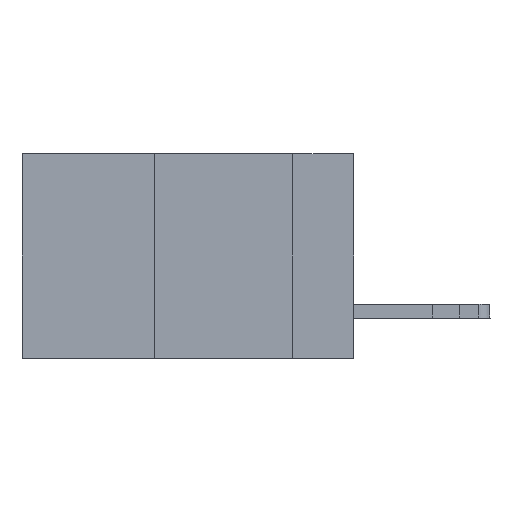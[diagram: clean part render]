
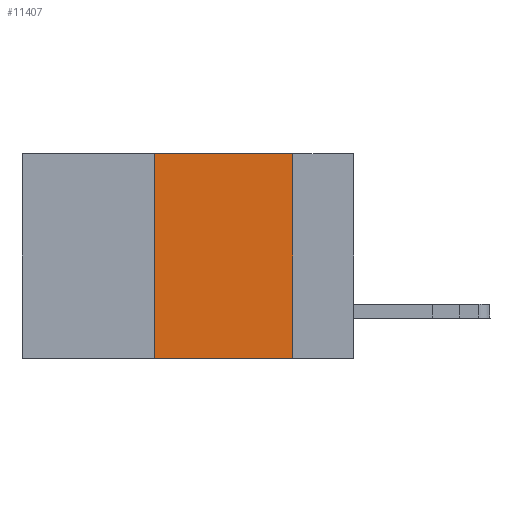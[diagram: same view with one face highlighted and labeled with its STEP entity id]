
A CAD part, left-side view. The second image highlights one B-rep face of the part: STEP entity #11407.
In plain terms, the highlighted planar face has unit normal (-1, 0, 0).
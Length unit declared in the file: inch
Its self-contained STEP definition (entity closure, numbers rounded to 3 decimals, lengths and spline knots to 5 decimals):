
#121 = DIRECTION ( 'NONE',  ( 0., 0., -1. ) ) ;
#979 = CARTESIAN_POINT ( 'NONE',  ( 0., 0.6, -0.37 ) ) ;
#1131 = EDGE_CURVE ( 'NONE', #9691, #8390, #1916, .T. ) ;
#1740 = DIRECTION ( 'NONE',  ( 0., -1., 0. ) ) ;
#1916 = LINE ( 'NONE', #7023, #8599 ) ;
#2719 = DIRECTION ( 'NONE',  ( 0., 0., 1. ) ) ;
#2920 = PLANE ( 'NONE',  #10691 ) ;
#3132 = ORIENTED_EDGE ( 'NONE', *, *, #3309, .F. ) ;
#3309 = EDGE_CURVE ( 'NONE', #19067, #4834, #12117, .T. ) ;
#3496 = VECTOR ( 'NONE', #2719, 39.37008 ) ;
#4452 = DIRECTION ( 'NONE',  ( 1., 0., 0. ) ) ;
#4834 = VERTEX_POINT ( 'NONE', #15654 ) ;
#5463 = CARTESIAN_POINT ( 'NONE',  ( 0., 0.11, -0.37 ) ) ;
#6012 = VECTOR ( 'NONE', #13217, 39.37008 ) ;
#6879 = EDGE_CURVE ( 'NONE', #19067, #8390, #14619, .T. ) ;
#7023 = CARTESIAN_POINT ( 'NONE',  ( 0., 0.11, 0. ) ) ;
#8390 = VERTEX_POINT ( 'NONE', #5463 ) ;
#8599 = VECTOR ( 'NONE', #121, 39.37008 ) ;
#9691 = VERTEX_POINT ( 'NONE', #17840 ) ;
#9805 = CARTESIAN_POINT ( 'NONE',  ( 0., 0.36, -0.37 ) ) ;
#10691 = AXIS2_PLACEMENT_3D ( 'NONE', #13629, #4452, #15168 ) ;
#10919 = EDGE_CURVE ( 'NONE', #4834, #9691, #11857, .T. ) ;
#11407 = ADVANCED_FACE ( 'NONE', ( #14451 ), #2920, .F. ) ;
#11857 = LINE ( 'NONE', #12451, #15463 ) ;
#11886 = CARTESIAN_POINT ( 'NONE',  ( 0., 0.36, 0. ) ) ;
#12117 = LINE ( 'NONE', #11886, #3496 ) ;
#12451 = CARTESIAN_POINT ( 'NONE',  ( 0., 0.6, 0. ) ) ;
#13217 = DIRECTION ( 'NONE',  ( 0., -1., 0. ) ) ;
#13629 = CARTESIAN_POINT ( 'NONE',  ( 0., 0.6, 0. ) ) ;
#14451 = FACE_OUTER_BOUND ( 'NONE', #17833, .T. ) ;
#14619 = LINE ( 'NONE', #979, #6012 ) ;
#15168 = DIRECTION ( 'NONE',  ( 0., 0., -1. ) ) ;
#15463 = VECTOR ( 'NONE', #1740, 39.37008 ) ;
#15654 = CARTESIAN_POINT ( 'NONE',  ( 0., 0.36, 0. ) ) ;
#17833 = EDGE_LOOP ( 'NONE', ( #18715, #18489, #3132, #19451 ) ) ;
#17840 = CARTESIAN_POINT ( 'NONE',  ( 0., 0.11, 0. ) ) ;
#18489 = ORIENTED_EDGE ( 'NONE', *, *, #10919, .F. ) ;
#18715 = ORIENTED_EDGE ( 'NONE', *, *, #1131, .F. ) ;
#19067 = VERTEX_POINT ( 'NONE', #9805 ) ;
#19451 = ORIENTED_EDGE ( 'NONE', *, *, #6879, .T. ) ;
